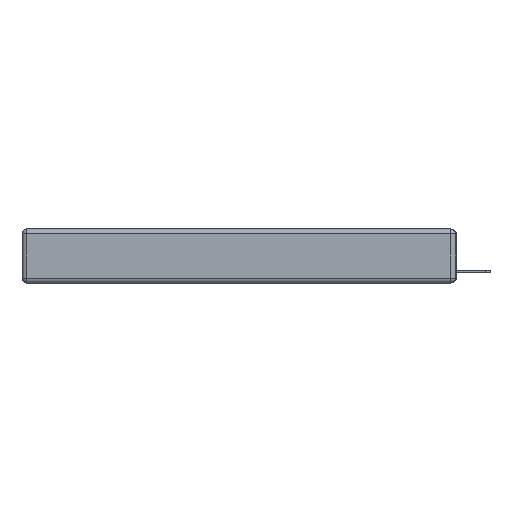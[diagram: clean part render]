
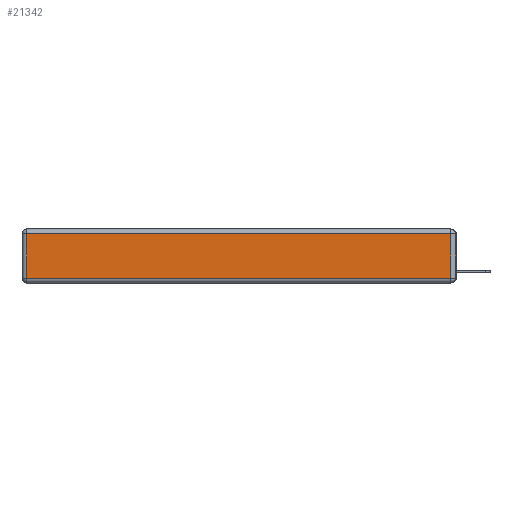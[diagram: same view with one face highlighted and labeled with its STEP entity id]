
A CAD part, left-side view. The second image highlights one B-rep face of the part: STEP entity #21342.
In plain terms, the highlighted planar face has unit normal (-1, 0, 0).
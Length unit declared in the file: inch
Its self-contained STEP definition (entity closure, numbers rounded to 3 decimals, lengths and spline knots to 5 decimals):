
#1395 = FACE_OUTER_BOUND ( 'NONE', #7564, .T. ) ;
#1532 = VERTEX_POINT ( 'NONE', #6787 ) ;
#2242 = CARTESIAN_POINT ( 'NONE',  ( 0., 0., -0.313 ) ) ;
#2906 = VERTEX_POINT ( 'NONE', #24369 ) ;
#3597 = LINE ( 'NONE', #3598, #13748 ) ;
#3598 = CARTESIAN_POINT ( 'NONE',  ( 0., 2.72, -0.343 ) ) ;
#3641 = EDGE_CURVE ( 'NONE', #12313, #24446, #4002, .T. ) ;
#4002 = LINE ( 'NONE', #14618, #24935 ) ;
#4151 = LINE ( 'NONE', #8654, #21274 ) ;
#5933 = ORIENTED_EDGE ( 'NONE', *, *, #16652, .T. ) ;
#6110 = LINE ( 'NONE', #2242, #19775 ) ;
#6787 = CARTESIAN_POINT ( 'NONE',  ( 0., 2.72, -0.313 ) ) ;
#7043 = EDGE_CURVE ( 'NONE', #24446, #2906, #4151, .T. ) ;
#7564 = EDGE_LOOP ( 'NONE', ( #11955, #16369, #12585, #5933 ) ) ;
#8294 = DIRECTION ( 'NONE',  ( -1., 0., 0. ) ) ;
#8654 = CARTESIAN_POINT ( 'NONE',  ( 0., 2.75, -0.03 ) ) ;
#10783 = DIRECTION ( 'NONE',  ( 0., 0., 1. ) ) ;
#11955 = ORIENTED_EDGE ( 'NONE', *, *, #22117, .T. ) ;
#12063 = AXIS2_PLACEMENT_3D ( 'NONE', #14510, #8294, #24718 ) ;
#12313 = VERTEX_POINT ( 'NONE', #14464 ) ;
#12585 = ORIENTED_EDGE ( 'NONE', *, *, #7043, .T. ) ;
#13045 = DIRECTION ( 'NONE',  ( 0., -1., 0. ) ) ;
#13520 = DIRECTION ( 'NONE',  ( 0., 0., -1. ) ) ;
#13748 = VECTOR ( 'NONE', #13520, 39.37008 ) ;
#14464 = CARTESIAN_POINT ( 'NONE',  ( 0., 0.03, -0.313 ) ) ;
#14510 = CARTESIAN_POINT ( 'NONE',  ( 0., 0., -0.343 ) ) ;
#14618 = CARTESIAN_POINT ( 'NONE',  ( 0., 0.03, -0.343 ) ) ;
#16369 = ORIENTED_EDGE ( 'NONE', *, *, #3641, .T. ) ;
#16652 = EDGE_CURVE ( 'NONE', #2906, #1532, #3597, .T. ) ;
#16880 = CARTESIAN_POINT ( 'NONE',  ( 0., 0.03, -0.03 ) ) ;
#19775 = VECTOR ( 'NONE', #13045, 39.37008 ) ;
#21274 = VECTOR ( 'NONE', #22958, 39.37008 ) ;
#21342 = ADVANCED_FACE ( 'NONE', ( #1395 ), #22668, .T. ) ;
#22117 = EDGE_CURVE ( 'NONE', #1532, #12313, #6110, .T. ) ;
#22668 = PLANE ( 'NONE',  #12063 ) ;
#22958 = DIRECTION ( 'NONE',  ( 0., 1., 0. ) ) ;
#24369 = CARTESIAN_POINT ( 'NONE',  ( 0., 2.72, -0.03 ) ) ;
#24446 = VERTEX_POINT ( 'NONE', #16880 ) ;
#24718 = DIRECTION ( 'NONE',  ( 0., 0., 1. ) ) ;
#24935 = VECTOR ( 'NONE', #10783, 39.37008 ) ;
